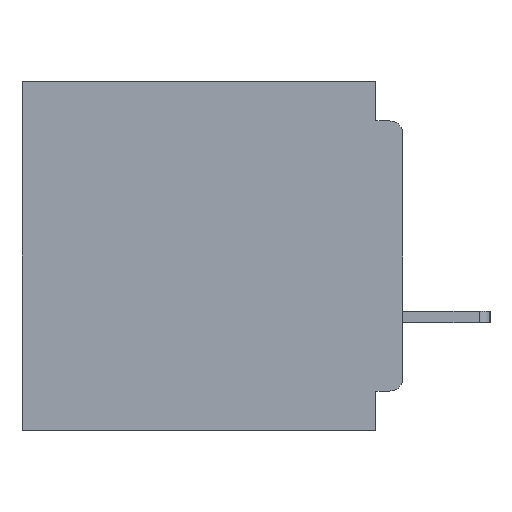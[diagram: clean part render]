
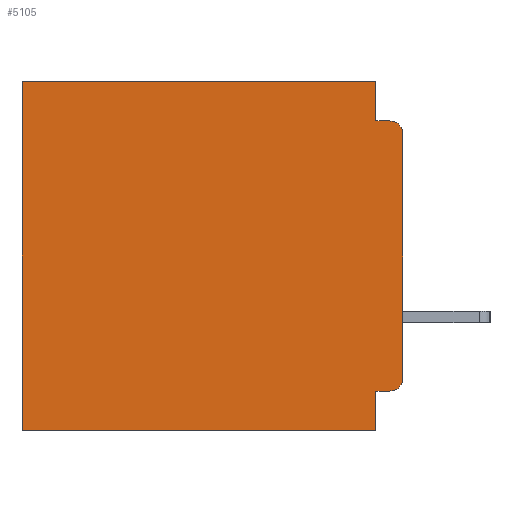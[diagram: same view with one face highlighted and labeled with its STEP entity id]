
A CAD part, left-side view. The second image highlights one B-rep face of the part: STEP entity #5105.
In plain terms, the highlighted planar face has unit normal (-1, 0, 0).
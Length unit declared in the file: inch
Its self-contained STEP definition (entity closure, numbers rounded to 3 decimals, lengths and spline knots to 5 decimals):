
#1525 = EDGE_CURVE ( 'NONE', #3434, #10345, #25867, .T. ) ;
#2370 = CARTESIAN_POINT ( 'NONE',  ( 0.3, 0.437, 0. ) ) ;
#3434 = VERTEX_POINT ( 'NONE', #36539 ) ;
#3704 = VERTEX_POINT ( 'NONE', #2370 ) ;
#3728 = AXIS2_PLACEMENT_3D ( 'NONE', #34881, #32689, #32345 ) ;
#3993 = DIRECTION ( 'NONE',  ( -1., 0., 0. ) ) ;
#5105 = ADVANCED_FACE ( 'NONE', ( #5441 ), #37102, .F. ) ;
#5441 = FACE_OUTER_BOUND ( 'NONE', #10489, .T. ) ;
#7302 = DIRECTION ( 'NONE',  ( 0., 0., -1. ) ) ;
#7410 = EDGE_CURVE ( 'NONE', #3704, #15994, #33573, .T. ) ;
#8095 = CARTESIAN_POINT ( 'NONE',  ( 0.3, 0.031, 0. ) ) ;
#8267 = CARTESIAN_POINT ( 'NONE',  ( 0.3, 0., -0.355 ) ) ;
#8522 = LINE ( 'NONE', #30088, #45084 ) ;
#10345 = VERTEX_POINT ( 'NONE', #36162 ) ;
#10406 = ORIENTED_EDGE ( 'NONE', *, *, #24728, .F. ) ;
#10489 = EDGE_LOOP ( 'NONE', ( #22502, #13528, #34795, #42795, #20045, #40681, #11736, #10406, #12690, #41865 ) ) ;
#11403 = EDGE_CURVE ( 'NONE', #27890, #32658, #36546, .T. ) ;
#11736 = ORIENTED_EDGE ( 'NONE', *, *, #25489, .F. ) ;
#12022 = DIRECTION ( 'NONE',  ( 0., 1., 0. ) ) ;
#12690 = ORIENTED_EDGE ( 'NONE', *, *, #1525, .F. ) ;
#13528 = ORIENTED_EDGE ( 'NONE', *, *, #24144, .T. ) ;
#14464 = CARTESIAN_POINT ( 'NONE',  ( 0.3, 0.031, -0.4 ) ) ;
#14574 = LINE ( 'NONE', #8095, #22945 ) ;
#14690 = VECTOR ( 'NONE', #33497, 39.37008 ) ;
#15324 = DIRECTION ( 'NONE',  ( 0., 0., -1. ) ) ;
#15974 = DIRECTION ( 'NONE',  ( -1., 0., 0. ) ) ;
#15994 = VERTEX_POINT ( 'NONE', #24477 ) ;
#17022 = VERTEX_POINT ( 'NONE', #43936 ) ;
#17792 = CARTESIAN_POINT ( 'NONE',  ( 0.3, 0., -0.045 ) ) ;
#19584 = DIRECTION ( 'NONE',  ( 0., 1., 0. ) ) ;
#20045 = ORIENTED_EDGE ( 'NONE', *, *, #31918, .T. ) ;
#20060 = CARTESIAN_POINT ( 'NONE',  ( 0.3, 0., -0.06 ) ) ;
#20915 = AXIS2_PLACEMENT_3D ( 'NONE', #37230, #15974, #40743 ) ;
#21211 = DIRECTION ( 'NONE',  ( 0., 1., 0. ) ) ;
#22051 = CARTESIAN_POINT ( 'NONE',  ( 0.3, 0.015, -0.045 ) ) ;
#22502 = ORIENTED_EDGE ( 'NONE', *, *, #45044, .F. ) ;
#22945 = VECTOR ( 'NONE', #36496, 39.37008 ) ;
#23568 = CIRCLE ( 'NONE', #20915, 0.015 ) ;
#24144 = EDGE_CURVE ( 'NONE', #36351, #32658, #45819, .T. ) ;
#24477 = CARTESIAN_POINT ( 'NONE',  ( 0.3, 0.437, -0.4 ) ) ;
#24728 = EDGE_CURVE ( 'NONE', #10345, #17022, #33610, .T. ) ;
#25409 = LINE ( 'NONE', #38812, #33697 ) ;
#25411 = CARTESIAN_POINT ( 'NONE',  ( 0.3, 0.015, -0.06 ) ) ;
#25489 = EDGE_CURVE ( 'NONE', #17022, #15994, #8522, .T. ) ;
#25557 = AXIS2_PLACEMENT_3D ( 'NONE', #25411, #3993, #28980 ) ;
#25771 = EDGE_CURVE ( 'NONE', #3434, #35597, #23568, .T. ) ;
#25867 = LINE ( 'NONE', #8267, #37499 ) ;
#26284 = CARTESIAN_POINT ( 'NONE',  ( 0.3, 0., -0.34 ) ) ;
#27890 = VERTEX_POINT ( 'NONE', #45925 ) ;
#28980 = DIRECTION ( 'NONE',  ( 0., 0., -1. ) ) ;
#28987 = LINE ( 'NONE', #33014, #36148 ) ;
#29942 = CARTESIAN_POINT ( 'NONE',  ( 0.3, 0.437, -0.4 ) ) ;
#30088 = CARTESIAN_POINT ( 'NONE',  ( 0.3, 0., -0.4 ) ) ;
#31577 = VERTEX_POINT ( 'NONE', #43872 ) ;
#31918 = EDGE_CURVE ( 'NONE', #31577, #3704, #25409, .T. ) ;
#32345 = DIRECTION ( 'NONE',  ( 0., 0., -1. ) ) ;
#32658 = VERTEX_POINT ( 'NONE', #22051 ) ;
#32689 = DIRECTION ( 'NONE',  ( 1., 0., 0. ) ) ;
#33014 = CARTESIAN_POINT ( 'NONE',  ( 0.3, 0., -0.4 ) ) ;
#33497 = DIRECTION ( 'NONE',  ( 0., 0., -1. ) ) ;
#33573 = LINE ( 'NONE', #29942, #14690 ) ;
#33610 = LINE ( 'NONE', #14464, #35816 ) ;
#33697 = VECTOR ( 'NONE', #21211, 39.37008 ) ;
#34795 = ORIENTED_EDGE ( 'NONE', *, *, #11403, .F. ) ;
#34881 = CARTESIAN_POINT ( 'NONE',  ( 0.3, 0., -0.4 ) ) ;
#35443 = DIRECTION ( 'NONE',  ( 0., -1., 0. ) ) ;
#35597 = VERTEX_POINT ( 'NONE', #26284 ) ;
#35816 = VECTOR ( 'NONE', #7302, 39.37008 ) ;
#36148 = VECTOR ( 'NONE', #15324, 39.37008 ) ;
#36162 = CARTESIAN_POINT ( 'NONE',  ( 0.3, 0.031, -0.355 ) ) ;
#36351 = VERTEX_POINT ( 'NONE', #20060 ) ;
#36496 = DIRECTION ( 'NONE',  ( 0., 0., -1. ) ) ;
#36539 = CARTESIAN_POINT ( 'NONE',  ( 0.3, 0.015, -0.355 ) ) ;
#36546 = LINE ( 'NONE', #17792, #45874 ) ;
#37102 = PLANE ( 'NONE',  #3728 ) ;
#37230 = CARTESIAN_POINT ( 'NONE',  ( 0.3, 0.015, -0.34 ) ) ;
#37499 = VECTOR ( 'NONE', #12022, 39.37008 ) ;
#38812 = CARTESIAN_POINT ( 'NONE',  ( 0.3, 0., 0. ) ) ;
#40681 = ORIENTED_EDGE ( 'NONE', *, *, #7410, .T. ) ;
#40743 = DIRECTION ( 'NONE',  ( 0., 0., -1. ) ) ;
#41218 = EDGE_CURVE ( 'NONE', #31577, #27890, #14574, .T. ) ;
#41865 = ORIENTED_EDGE ( 'NONE', *, *, #25771, .T. ) ;
#42795 = ORIENTED_EDGE ( 'NONE', *, *, #41218, .F. ) ;
#43872 = CARTESIAN_POINT ( 'NONE',  ( 0.3, 0.031, 0. ) ) ;
#43936 = CARTESIAN_POINT ( 'NONE',  ( 0.3, 0.031, -0.4 ) ) ;
#45044 = EDGE_CURVE ( 'NONE', #36351, #35597, #28987, .T. ) ;
#45084 = VECTOR ( 'NONE', #19584, 39.37008 ) ;
#45819 = CIRCLE ( 'NONE', #25557, 0.015 ) ;
#45874 = VECTOR ( 'NONE', #35443, 39.37008 ) ;
#45925 = CARTESIAN_POINT ( 'NONE',  ( 0.3, 0.031, -0.045 ) ) ;
